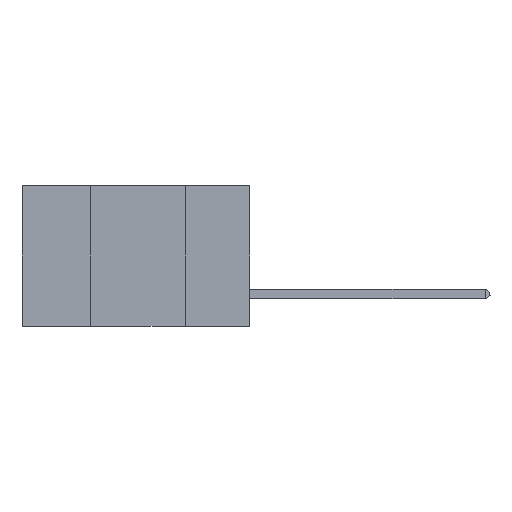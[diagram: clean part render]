
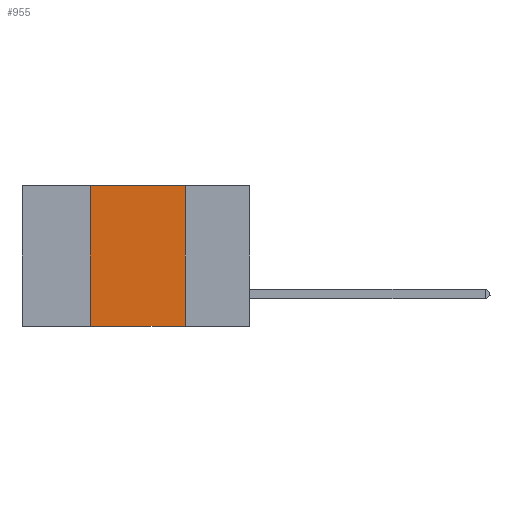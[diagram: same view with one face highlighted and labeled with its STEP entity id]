
A CAD part, left-side view. The second image highlights one B-rep face of the part: STEP entity #955.
In plain terms, the highlighted planar face has unit normal (-1, 0, 0).
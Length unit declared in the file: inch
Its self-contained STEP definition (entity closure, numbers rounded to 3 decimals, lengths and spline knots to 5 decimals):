
#256 = EDGE_CURVE ( 'NONE', #6410, #5320, #9407, .T. ) ;
#903 = VECTOR ( 'NONE', #4741, 39.37008 ) ;
#955 = ADVANCED_FACE ( 'NONE', ( #11779 ), #1442, .F. ) ;
#1079 = CARTESIAN_POINT ( 'NONE',  ( 0., 0.17, -0.37 ) ) ;
#1442 = PLANE ( 'NONE',  #1818 ) ;
#1654 = EDGE_CURVE ( 'NONE', #6410, #11892, #2726, .T. ) ;
#1701 = EDGE_CURVE ( 'NONE', #8377, #11892, #2578, .T. ) ;
#1818 = AXIS2_PLACEMENT_3D ( 'NONE', #4830, #13438, #9131 ) ;
#1999 = ORIENTED_EDGE ( 'NONE', *, *, #1654, .T. ) ;
#2107 = EDGE_CURVE ( 'NONE', #5320, #8377, #7224, .T. ) ;
#2481 = ORIENTED_EDGE ( 'NONE', *, *, #1701, .F. ) ;
#2578 = LINE ( 'NONE', #8069, #5880 ) ;
#2726 = LINE ( 'NONE', #11135, #903 ) ;
#3328 = DIRECTION ( 'NONE',  ( 0., -1., 0. ) ) ;
#4483 = EDGE_LOOP ( 'NONE', ( #2481, #7394, #10772, #1999 ) ) ;
#4741 = DIRECTION ( 'NONE',  ( 0., -1., 0. ) ) ;
#4830 = CARTESIAN_POINT ( 'NONE',  ( 0., 0.6, 0. ) ) ;
#5097 = CARTESIAN_POINT ( 'NONE',  ( 0., 0.42, -0.37 ) ) ;
#5320 = VERTEX_POINT ( 'NONE', #5490 ) ;
#5490 = CARTESIAN_POINT ( 'NONE',  ( 0., 0.42, 0. ) ) ;
#5871 = DIRECTION ( 'NONE',  ( 0., 0., -1. ) ) ;
#5880 = VECTOR ( 'NONE', #5871, 39.37008 ) ;
#6410 = VERTEX_POINT ( 'NONE', #5097 ) ;
#7224 = LINE ( 'NONE', #8820, #9048 ) ;
#7394 = ORIENTED_EDGE ( 'NONE', *, *, #2107, .F. ) ;
#8069 = CARTESIAN_POINT ( 'NONE',  ( 0., 0.17, 0. ) ) ;
#8377 = VERTEX_POINT ( 'NONE', #8720 ) ;
#8720 = CARTESIAN_POINT ( 'NONE',  ( 0., 0.17, 0. ) ) ;
#8820 = CARTESIAN_POINT ( 'NONE',  ( 0., 0.6, 0. ) ) ;
#9048 = VECTOR ( 'NONE', #3328, 39.37008 ) ;
#9131 = DIRECTION ( 'NONE',  ( 0., 0., -1. ) ) ;
#9407 = LINE ( 'NONE', #12783, #12410 ) ;
#10772 = ORIENTED_EDGE ( 'NONE', *, *, #256, .F. ) ;
#11135 = CARTESIAN_POINT ( 'NONE',  ( 0., 0.6, -0.37 ) ) ;
#11779 = FACE_OUTER_BOUND ( 'NONE', #4483, .T. ) ;
#11892 = VERTEX_POINT ( 'NONE', #1079 ) ;
#12410 = VECTOR ( 'NONE', #12683, 39.37008 ) ;
#12683 = DIRECTION ( 'NONE',  ( 0., 0., 1. ) ) ;
#12783 = CARTESIAN_POINT ( 'NONE',  ( 0., 0.42, 0. ) ) ;
#13438 = DIRECTION ( 'NONE',  ( 1., 0., 0. ) ) ;
